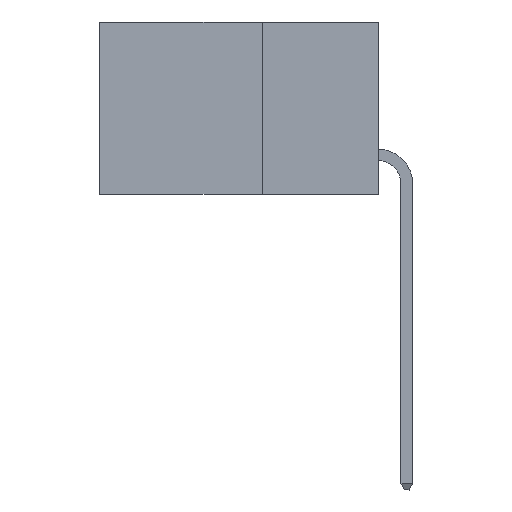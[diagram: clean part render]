
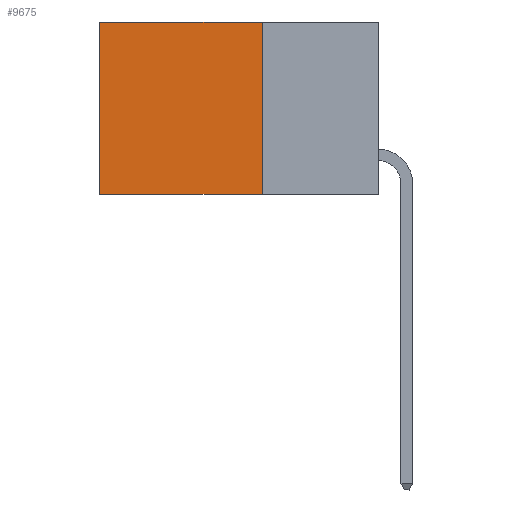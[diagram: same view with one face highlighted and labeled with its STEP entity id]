
A CAD part, left-side view. The second image highlights one B-rep face of the part: STEP entity #9675.
In plain terms, the highlighted planar face has unit normal (-1, 0, 0).
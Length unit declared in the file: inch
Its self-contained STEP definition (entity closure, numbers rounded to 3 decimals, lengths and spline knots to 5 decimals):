
#158 = EDGE_CURVE ( 'NONE', #7678, #5508, #6335, .T. ) ;
#180 = DIRECTION ( 'NONE',  ( 0., 0., -1. ) ) ;
#514 = VECTOR ( 'NONE', #4658, 39.37008 ) ;
#646 = PLANE ( 'NONE',  #2367 ) ;
#674 = LINE ( 'NONE', #10301, #514 ) ;
#1277 = CARTESIAN_POINT ( 'NONE',  ( 0.2615, 0.25, -0.37 ) ) ;
#2251 = VECTOR ( 'NONE', #7862, 39.37008 ) ;
#2367 = AXIS2_PLACEMENT_3D ( 'NONE', #7087, #3860, #8097 ) ;
#2865 = EDGE_CURVE ( 'NONE', #5508, #2992, #8802, .T. ) ;
#2992 = VERTEX_POINT ( 'NONE', #9115 ) ;
#3670 = CARTESIAN_POINT ( 'NONE',  ( 0.2615, 0.6, 0. ) ) ;
#3860 = DIRECTION ( 'NONE',  ( 1., 0., 0. ) ) ;
#4658 = DIRECTION ( 'NONE',  ( 0., 0., -1. ) ) ;
#4662 = CARTESIAN_POINT ( 'NONE',  ( 0.2615, 0.25, 0. ) ) ;
#5448 = EDGE_CURVE ( 'NONE', #5752, #2992, #7590, .T. ) ;
#5508 = VERTEX_POINT ( 'NONE', #3670 ) ;
#5752 = VERTEX_POINT ( 'NONE', #8156 ) ;
#6101 = DIRECTION ( 'NONE',  ( 0., 1., 0. ) ) ;
#6335 = LINE ( 'NONE', #4662, #2251 ) ;
#6375 = CARTESIAN_POINT ( 'NONE',  ( 0.2615, 0.6, -0.37 ) ) ;
#7087 = CARTESIAN_POINT ( 'NONE',  ( 0.2615, 0.25, -0.37 ) ) ;
#7103 = ORIENTED_EDGE ( 'NONE', *, *, #9871, .F. ) ;
#7513 = VECTOR ( 'NONE', #6101, 39.37008 ) ;
#7590 = LINE ( 'NONE', #1277, #7513 ) ;
#7677 = ORIENTED_EDGE ( 'NONE', *, *, #2865, .T. ) ;
#7678 = VERTEX_POINT ( 'NONE', #7716 ) ;
#7716 = CARTESIAN_POINT ( 'NONE',  ( 0.2615, 0.25, 0. ) ) ;
#7720 = VECTOR ( 'NONE', #180, 39.37008 ) ;
#7829 = FACE_OUTER_BOUND ( 'NONE', #9994, .T. ) ;
#7862 = DIRECTION ( 'NONE',  ( 0., 1., 0. ) ) ;
#8097 = DIRECTION ( 'NONE',  ( 0., 0., -1. ) ) ;
#8156 = CARTESIAN_POINT ( 'NONE',  ( 0.2615, 0.25, -0.37 ) ) ;
#8660 = ORIENTED_EDGE ( 'NONE', *, *, #158, .T. ) ;
#8802 = LINE ( 'NONE', #6375, #7720 ) ;
#8935 = ORIENTED_EDGE ( 'NONE', *, *, #5448, .F. ) ;
#9115 = CARTESIAN_POINT ( 'NONE',  ( 0.2615, 0.6, -0.37 ) ) ;
#9675 = ADVANCED_FACE ( 'NONE', ( #7829 ), #646, .F. ) ;
#9871 = EDGE_CURVE ( 'NONE', #7678, #5752, #674, .T. ) ;
#9994 = EDGE_LOOP ( 'NONE', ( #7677, #8935, #7103, #8660 ) ) ;
#10301 = CARTESIAN_POINT ( 'NONE',  ( 0.2615, 0.25, -0.37 ) ) ;
